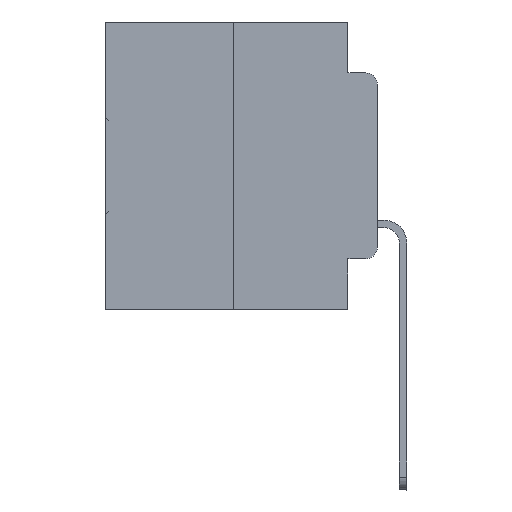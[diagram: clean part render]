
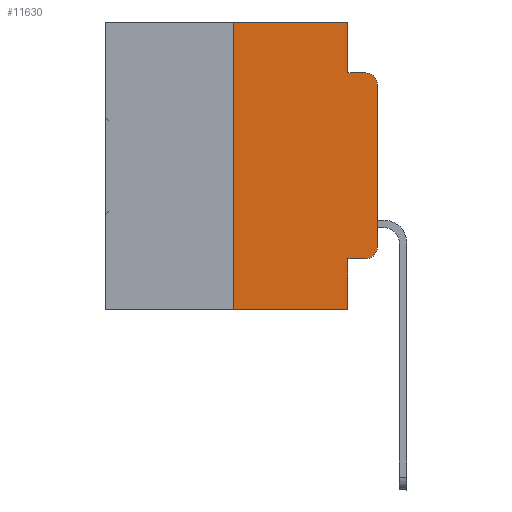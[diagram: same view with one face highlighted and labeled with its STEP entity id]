
A CAD part, left-side view. The second image highlights one B-rep face of the part: STEP entity #11630.
In plain terms, the highlighted planar face has unit normal (-1, 0, 0).
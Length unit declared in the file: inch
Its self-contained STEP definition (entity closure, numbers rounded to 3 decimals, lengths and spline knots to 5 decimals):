
#712 = CARTESIAN_POINT ( 'NONE',  ( 0., 0.051, -0.4115 ) ) ;
#811 = CARTESIAN_POINT ( 'NONE',  ( 0., 0.051, -0.4115 ) ) ;
#919 = VERTEX_POINT ( 'NONE', #5280 ) ;
#1355 = ORIENTED_EDGE ( 'NONE', *, *, #21396, .F. ) ;
#1374 = ORIENTED_EDGE ( 'NONE', *, *, #19701, .F. ) ;
#1453 = CARTESIAN_POINT ( 'NONE',  ( 0., 0.02, -0.0885 ) ) ;
#1855 = VERTEX_POINT ( 'NONE', #8370 ) ;
#2307 = VERTEX_POINT ( 'NONE', #30330 ) ;
#2778 = ORIENTED_EDGE ( 'NONE', *, *, #30311, .F. ) ;
#3769 = EDGE_CURVE ( 'NONE', #11085, #17948, #12999, .T. ) ;
#3935 = ORIENTED_EDGE ( 'NONE', *, *, #12062, .T. ) ;
#4138 = DIRECTION ( 'NONE',  ( 0., -1., 0. ) ) ;
#4414 = AXIS2_PLACEMENT_3D ( 'NONE', #8012, #22167, #17345 ) ;
#4662 = DIRECTION ( 'NONE',  ( 0., -1., 0. ) ) ;
#5089 = LINE ( 'NONE', #19714, #5962 ) ;
#5280 = CARTESIAN_POINT ( 'NONE',  ( 0., 0.051, 0. ) ) ;
#5299 = VERTEX_POINT ( 'NONE', #17322 ) ;
#5962 = VECTOR ( 'NONE', #7973, 39.37008 ) ;
#6037 = ORIENTED_EDGE ( 'NONE', *, *, #13572, .T. ) ;
#6717 = CARTESIAN_POINT ( 'NONE',  ( 0., 0.051, 0. ) ) ;
#6734 = LINE ( 'NONE', #21350, #23004 ) ;
#6759 = EDGE_CURVE ( 'NONE', #17948, #1855, #27310, .T. ) ;
#6862 = LINE ( 'NONE', #20834, #22102 ) ;
#7187 = CARTESIAN_POINT ( 'NONE',  ( 0., 0.02, -0.4115 ) ) ;
#7877 = DIRECTION ( 'NONE',  ( -1., 0., 0. ) ) ;
#7973 = DIRECTION ( 'NONE',  ( 0., -1., 0. ) ) ;
#8012 = CARTESIAN_POINT ( 'NONE',  ( 0., 0.473, 0. ) ) ;
#8370 = CARTESIAN_POINT ( 'NONE',  ( 0., 0., -0.3915 ) ) ;
#8400 = ORIENTED_EDGE ( 'NONE', *, *, #3769, .T. ) ;
#8662 = DIRECTION ( 'NONE',  ( 0., 0., 1. ) ) ;
#11085 = VERTEX_POINT ( 'NONE', #712 ) ;
#11630 = ADVANCED_FACE ( 'NONE', ( #20367 ), #25039, .F. ) ;
#12034 = VERTEX_POINT ( 'NONE', #24845 ) ;
#12062 = EDGE_CURVE ( 'NONE', #12034, #17957, #5089, .T. ) ;
#12999 = LINE ( 'NONE', #811, #14759 ) ;
#13049 = LINE ( 'NONE', #27836, #29078 ) ;
#13087 = DIRECTION ( 'NONE',  ( 0., 0., 1. ) ) ;
#13108 = DIRECTION ( 'NONE',  ( 0., 0., -1. ) ) ;
#13249 = CIRCLE ( 'NONE', #15300, 0.02 ) ;
#13572 = EDGE_CURVE ( 'NONE', #25217, #31681, #13249, .T. ) ;
#14759 = VECTOR ( 'NONE', #22635, 39.37008 ) ;
#14993 = AXIS2_PLACEMENT_3D ( 'NONE', #29887, #7877, #17834 ) ;
#15300 = AXIS2_PLACEMENT_3D ( 'NONE', #28853, #21299, #21611 ) ;
#15628 = DIRECTION ( 'NONE',  ( 0., 0., -1. ) ) ;
#16883 = CARTESIAN_POINT ( 'NONE',  ( 0., 0.051, -0.0885 ) ) ;
#17322 = CARTESIAN_POINT ( 'NONE',  ( 0., 0.25, 0. ) ) ;
#17345 = DIRECTION ( 'NONE',  ( 0., 0., -1. ) ) ;
#17434 = CARTESIAN_POINT ( 'NONE',  ( 0., 0., -0.1085 ) ) ;
#17791 = EDGE_CURVE ( 'NONE', #5299, #919, #6862, .T. ) ;
#17834 = DIRECTION ( 'NONE',  ( 0., 0., -1. ) ) ;
#17948 = VERTEX_POINT ( 'NONE', #7187 ) ;
#17957 = VERTEX_POINT ( 'NONE', #30121 ) ;
#18559 = VECTOR ( 'NONE', #13087, 39.37008 ) ;
#19701 = EDGE_CURVE ( 'NONE', #919, #2307, #13049, .T. ) ;
#19714 = CARTESIAN_POINT ( 'NONE',  ( 0., 0.473, -0.5 ) ) ;
#19769 = EDGE_CURVE ( 'NONE', #2307, #31681, #26518, .T. ) ;
#20367 = FACE_OUTER_BOUND ( 'NONE', #26612, .T. ) ;
#20834 = CARTESIAN_POINT ( 'NONE',  ( 0., 0.473, 0. ) ) ;
#21299 = DIRECTION ( 'NONE',  ( -1., 0., 0. ) ) ;
#21350 = CARTESIAN_POINT ( 'NONE',  ( 0., 0.25, 0. ) ) ;
#21396 = EDGE_CURVE ( 'NONE', #12034, #5299, #6734, .T. ) ;
#21611 = DIRECTION ( 'NONE',  ( 0., 0., -1. ) ) ;
#22102 = VECTOR ( 'NONE', #4138, 39.37008 ) ;
#22167 = DIRECTION ( 'NONE',  ( 1., 0., 0. ) ) ;
#22635 = DIRECTION ( 'NONE',  ( 0., -1., 0. ) ) ;
#23004 = VECTOR ( 'NONE', #8662, 39.37008 ) ;
#23043 = CARTESIAN_POINT ( 'NONE',  ( 0., 0., 0. ) ) ;
#23555 = ORIENTED_EDGE ( 'NONE', *, *, #17791, .F. ) ;
#24211 = ORIENTED_EDGE ( 'NONE', *, *, #26524, .T. ) ;
#24845 = CARTESIAN_POINT ( 'NONE',  ( 0., 0.25, -0.5 ) ) ;
#25039 = PLANE ( 'NONE',  #4414 ) ;
#25104 = ORIENTED_EDGE ( 'NONE', *, *, #6759, .T. ) ;
#25217 = VERTEX_POINT ( 'NONE', #17434 ) ;
#25338 = VECTOR ( 'NONE', #13108, 39.37008 ) ;
#26518 = LINE ( 'NONE', #16883, #27543 ) ;
#26524 = EDGE_CURVE ( 'NONE', #1855, #25217, #28167, .T. ) ;
#26612 = EDGE_LOOP ( 'NONE', ( #24211, #6037, #29453, #1374, #23555, #1355, #3935, #2778, #8400, #25104 ) ) ;
#26782 = LINE ( 'NONE', #6717, #25338 ) ;
#27310 = CIRCLE ( 'NONE', #14993, 0.02 ) ;
#27543 = VECTOR ( 'NONE', #4662, 39.37008 ) ;
#27836 = CARTESIAN_POINT ( 'NONE',  ( 0., 0.051, 0. ) ) ;
#28167 = LINE ( 'NONE', #23043, #18559 ) ;
#28853 = CARTESIAN_POINT ( 'NONE',  ( 0., 0.02, -0.1085 ) ) ;
#29078 = VECTOR ( 'NONE', #15628, 39.37008 ) ;
#29453 = ORIENTED_EDGE ( 'NONE', *, *, #19769, .F. ) ;
#29887 = CARTESIAN_POINT ( 'NONE',  ( 0., 0.02, -0.3915 ) ) ;
#30121 = CARTESIAN_POINT ( 'NONE',  ( 0., 0.051, -0.5 ) ) ;
#30311 = EDGE_CURVE ( 'NONE', #11085, #17957, #26782, .T. ) ;
#30330 = CARTESIAN_POINT ( 'NONE',  ( 0., 0.051, -0.0885 ) ) ;
#31681 = VERTEX_POINT ( 'NONE', #1453 ) ;
